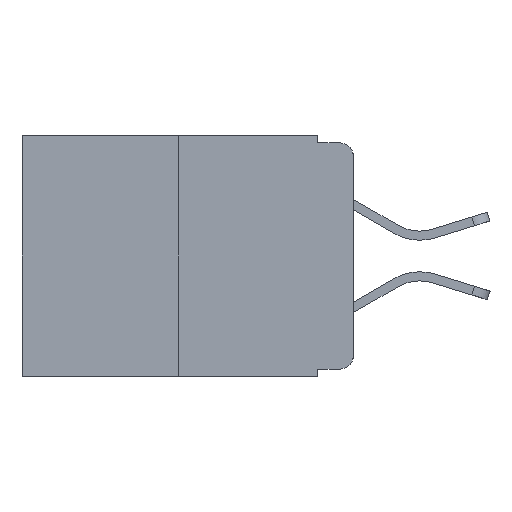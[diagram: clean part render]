
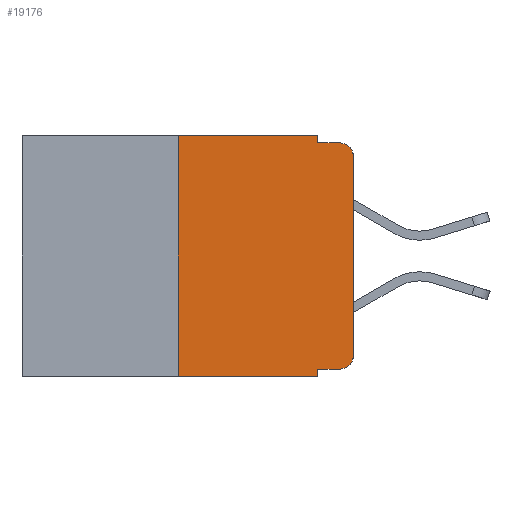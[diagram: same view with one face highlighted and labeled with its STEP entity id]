
A CAD part, left-side view. The second image highlights one B-rep face of the part: STEP entity #19176.
In plain terms, the highlighted planar face has unit normal (-1, 0, 0).
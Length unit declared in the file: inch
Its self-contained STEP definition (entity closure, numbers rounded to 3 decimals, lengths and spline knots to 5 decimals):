
#194 = DIRECTION ( 'NONE',  ( 0., 0., -1. ) ) ;
#264 = VERTEX_POINT ( 'NONE', #20568 ) ;
#276 = CIRCLE ( 'NONE', #3209, 0.02 ) ;
#498 = DIRECTION ( 'NONE',  ( 0., -1., 0. ) ) ;
#555 = ORIENTED_EDGE ( 'NONE', *, *, #2959, .T. ) ;
#682 = CARTESIAN_POINT ( 'NONE',  ( 0., 0.051, -0.01 ) ) ;
#741 = CARTESIAN_POINT ( 'NONE',  ( 0., 0.473, 0. ) ) ;
#1174 = CARTESIAN_POINT ( 'NONE',  ( 0., 0.051, -0.343 ) ) ;
#1381 = DIRECTION ( 'NONE',  ( 0., 0., 1. ) ) ;
#1500 = VECTOR ( 'NONE', #13118, 39.37008 ) ;
#1591 = LINE ( 'NONE', #8703, #6752 ) ;
#1716 = AXIS2_PLACEMENT_3D ( 'NONE', #19270, #10143, #13671 ) ;
#1921 = VECTOR ( 'NONE', #194, 39.37008 ) ;
#1924 = DIRECTION ( 'NONE',  ( 0., 0., -1. ) ) ;
#2959 = EDGE_CURVE ( 'NONE', #8735, #20620, #11468, .T. ) ;
#3209 = AXIS2_PLACEMENT_3D ( 'NONE', #20926, #12149, #19000 ) ;
#3272 = ORIENTED_EDGE ( 'NONE', *, *, #5222, .F. ) ;
#3952 = DIRECTION ( 'NONE',  ( 0., -1., 0. ) ) ;
#4916 = VERTEX_POINT ( 'NONE', #6051 ) ;
#5021 = EDGE_CURVE ( 'NONE', #4916, #13387, #1591, .T. ) ;
#5222 = EDGE_CURVE ( 'NONE', #8735, #16066, #12335, .T. ) ;
#5576 = ORIENTED_EDGE ( 'NONE', *, *, #9340, .F. ) ;
#5906 = LINE ( 'NONE', #13220, #1500 ) ;
#6051 = CARTESIAN_POINT ( 'NONE',  ( 0., 0., -0.313 ) ) ;
#6145 = VERTEX_POINT ( 'NONE', #10659 ) ;
#6752 = VECTOR ( 'NONE', #1381, 39.37008 ) ;
#6825 = FACE_OUTER_BOUND ( 'NONE', #7394, .T. ) ;
#7306 = CARTESIAN_POINT ( 'NONE',  ( 0., 0.02, -0.333 ) ) ;
#7310 = CARTESIAN_POINT ( 'NONE',  ( 0., 0.25, -0.343 ) ) ;
#7357 = ORIENTED_EDGE ( 'NONE', *, *, #12742, .T. ) ;
#7375 = VERTEX_POINT ( 'NONE', #17631 ) ;
#7394 = EDGE_LOOP ( 'NONE', ( #10548, #9768, #17599, #5576, #9668, #8220, #16607, #3272, #555, #7357 ) ) ;
#7861 = EDGE_CURVE ( 'NONE', #14856, #16066, #14283, .T. ) ;
#8220 = ORIENTED_EDGE ( 'NONE', *, *, #10682, .F. ) ;
#8608 = VECTOR ( 'NONE', #12565, 39.37008 ) ;
#8703 = CARTESIAN_POINT ( 'NONE',  ( 0., 0., 0. ) ) ;
#8735 = VERTEX_POINT ( 'NONE', #11004 ) ;
#9340 = EDGE_CURVE ( 'NONE', #10177, #264, #18611, .T. ) ;
#9538 = CIRCLE ( 'NONE', #12445, 0.02 ) ;
#9656 = CARTESIAN_POINT ( 'NONE',  ( 0., 0.051, -0.333 ) ) ;
#9668 = ORIENTED_EDGE ( 'NONE', *, *, #11119, .F. ) ;
#9768 = ORIENTED_EDGE ( 'NONE', *, *, #10697, .T. ) ;
#10143 = DIRECTION ( 'NONE',  ( 1., 0., 0. ) ) ;
#10177 = VERTEX_POINT ( 'NONE', #22500 ) ;
#10548 = ORIENTED_EDGE ( 'NONE', *, *, #5021, .T. ) ;
#10659 = CARTESIAN_POINT ( 'NONE',  ( 0., 0.25, 0. ) ) ;
#10682 = EDGE_CURVE ( 'NONE', #14856, #6145, #5906, .T. ) ;
#10697 = EDGE_CURVE ( 'NONE', #13387, #7375, #9538, .T. ) ;
#11004 = CARTESIAN_POINT ( 'NONE',  ( 0., 0.051, -0.333 ) ) ;
#11119 = EDGE_CURVE ( 'NONE', #6145, #10177, #18326, .T. ) ;
#11468 = LINE ( 'NONE', #9656, #19795 ) ;
#12149 = DIRECTION ( 'NONE',  ( -1., 0., 0. ) ) ;
#12325 = CARTESIAN_POINT ( 'NONE',  ( 0., 0.051, 0. ) ) ;
#12335 = LINE ( 'NONE', #12672, #16212 ) ;
#12445 = AXIS2_PLACEMENT_3D ( 'NONE', #21781, #20070, #19842 ) ;
#12565 = DIRECTION ( 'NONE',  ( 0., -1., 0. ) ) ;
#12584 = CARTESIAN_POINT ( 'NONE',  ( 0., 0.473, -0.343 ) ) ;
#12672 = CARTESIAN_POINT ( 'NONE',  ( 0., 0.051, 0. ) ) ;
#12742 = EDGE_CURVE ( 'NONE', #20620, #4916, #276, .T. ) ;
#13118 = DIRECTION ( 'NONE',  ( 0., 0., 1. ) ) ;
#13220 = CARTESIAN_POINT ( 'NONE',  ( 0., 0.25, 0. ) ) ;
#13387 = VERTEX_POINT ( 'NONE', #15200 ) ;
#13671 = DIRECTION ( 'NONE',  ( 0., 0., -1. ) ) ;
#14283 = LINE ( 'NONE', #12584, #17707 ) ;
#14856 = VERTEX_POINT ( 'NONE', #7310 ) ;
#15200 = CARTESIAN_POINT ( 'NONE',  ( 0., 0., -0.03 ) ) ;
#16066 = VERTEX_POINT ( 'NONE', #1174 ) ;
#16212 = VECTOR ( 'NONE', #1924, 39.37008 ) ;
#16336 = LINE ( 'NONE', #682, #8608 ) ;
#16607 = ORIENTED_EDGE ( 'NONE', *, *, #7861, .T. ) ;
#17314 = PLANE ( 'NONE',  #1716 ) ;
#17599 = ORIENTED_EDGE ( 'NONE', *, *, #22437, .F. ) ;
#17631 = CARTESIAN_POINT ( 'NONE',  ( 0., 0.02, -0.01 ) ) ;
#17707 = VECTOR ( 'NONE', #21022, 39.37008 ) ;
#17790 = VECTOR ( 'NONE', #3952, 39.37008 ) ;
#18326 = LINE ( 'NONE', #741, #17790 ) ;
#18611 = LINE ( 'NONE', #12325, #1921 ) ;
#19000 = DIRECTION ( 'NONE',  ( 0., 0., -1. ) ) ;
#19176 = ADVANCED_FACE ( 'NONE', ( #6825 ), #17314, .F. ) ;
#19270 = CARTESIAN_POINT ( 'NONE',  ( 0., 0.473, 0. ) ) ;
#19795 = VECTOR ( 'NONE', #498, 39.37008 ) ;
#19842 = DIRECTION ( 'NONE',  ( 0., 0., -1. ) ) ;
#20070 = DIRECTION ( 'NONE',  ( -1., 0., 0. ) ) ;
#20568 = CARTESIAN_POINT ( 'NONE',  ( 0., 0.051, -0.01 ) ) ;
#20620 = VERTEX_POINT ( 'NONE', #7306 ) ;
#20926 = CARTESIAN_POINT ( 'NONE',  ( 0., 0.02, -0.313 ) ) ;
#21022 = DIRECTION ( 'NONE',  ( 0., -1., 0. ) ) ;
#21781 = CARTESIAN_POINT ( 'NONE',  ( 0., 0.02, -0.03 ) ) ;
#22437 = EDGE_CURVE ( 'NONE', #264, #7375, #16336, .T. ) ;
#22500 = CARTESIAN_POINT ( 'NONE',  ( 0., 0.051, 0. ) ) ;
